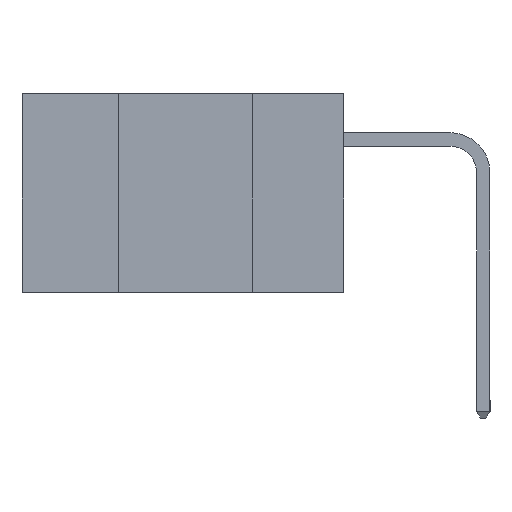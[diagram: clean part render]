
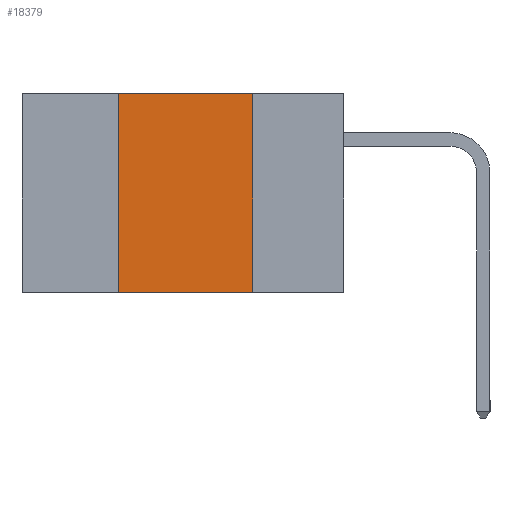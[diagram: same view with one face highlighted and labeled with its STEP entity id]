
A CAD part, left-side view. The second image highlights one B-rep face of the part: STEP entity #18379.
In plain terms, the highlighted planar face has unit normal (-1, 0, 0).
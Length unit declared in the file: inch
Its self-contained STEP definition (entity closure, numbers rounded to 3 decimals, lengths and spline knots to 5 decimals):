
#457 = DIRECTION ( 'NONE',  ( 0., 0., -1. ) ) ;
#1163 = CARTESIAN_POINT ( 'NONE',  ( 0., 0.42, -0.37 ) ) ;
#1395 = CARTESIAN_POINT ( 'NONE',  ( 0., 0.6, 0. ) ) ;
#1983 = ORIENTED_EDGE ( 'NONE', *, *, #7339, .T. ) ;
#4529 = DIRECTION ( 'NONE',  ( 0., -1., 0. ) ) ;
#4716 = DIRECTION ( 'NONE',  ( 0., -1., 0. ) ) ;
#5284 = CARTESIAN_POINT ( 'NONE',  ( 0., 0.6, -0.37 ) ) ;
#5469 = LINE ( 'NONE', #24870, #10307 ) ;
#5555 = ORIENTED_EDGE ( 'NONE', *, *, #8697, .F. ) ;
#6281 = VERTEX_POINT ( 'NONE', #24155 ) ;
#6349 = VERTEX_POINT ( 'NONE', #22588 ) ;
#7238 = FACE_OUTER_BOUND ( 'NONE', #24895, .T. ) ;
#7339 = EDGE_CURVE ( 'NONE', #10685, #6281, #23812, .T. ) ;
#8626 = LINE ( 'NONE', #16956, #13447 ) ;
#8697 = EDGE_CURVE ( 'NONE', #10685, #20961, #18172, .T. ) ;
#10307 = VECTOR ( 'NONE', #4716, 39.37008 ) ;
#10392 = ORIENTED_EDGE ( 'NONE', *, *, #21307, .F. ) ;
#10685 = VERTEX_POINT ( 'NONE', #23984 ) ;
#11809 = DIRECTION ( 'NONE',  ( 0., 0., -1. ) ) ;
#12139 = VECTOR ( 'NONE', #21651, 39.37008 ) ;
#13447 = VECTOR ( 'NONE', #457, 39.37008 ) ;
#16420 = EDGE_CURVE ( 'NONE', #6349, #6281, #8626, .T. ) ;
#16459 = ORIENTED_EDGE ( 'NONE', *, *, #16420, .F. ) ;
#16956 = CARTESIAN_POINT ( 'NONE',  ( 0., 0.17, -0.37 ) ) ;
#18172 = LINE ( 'NONE', #1163, #12139 ) ;
#18379 = ADVANCED_FACE ( 'NONE', ( #7238 ), #21860, .F. ) ;
#18518 = VECTOR ( 'NONE', #4529, 39.37008 ) ;
#20961 = VERTEX_POINT ( 'NONE', #23855 ) ;
#21307 = EDGE_CURVE ( 'NONE', #20961, #6349, #5469, .T. ) ;
#21651 = DIRECTION ( 'NONE',  ( 0., 0., 1. ) ) ;
#21860 = PLANE ( 'NONE',  #24963 ) ;
#22588 = CARTESIAN_POINT ( 'NONE',  ( 0., 0.17, 0. ) ) ;
#23812 = LINE ( 'NONE', #5284, #18518 ) ;
#23844 = DIRECTION ( 'NONE',  ( 1., 0., 0. ) ) ;
#23855 = CARTESIAN_POINT ( 'NONE',  ( 0., 0.42, 0. ) ) ;
#23984 = CARTESIAN_POINT ( 'NONE',  ( 0., 0.42, -0.37 ) ) ;
#24155 = CARTESIAN_POINT ( 'NONE',  ( 0., 0.17, -0.37 ) ) ;
#24870 = CARTESIAN_POINT ( 'NONE',  ( 0., 0.6, 0. ) ) ;
#24895 = EDGE_LOOP ( 'NONE', ( #16459, #10392, #5555, #1983 ) ) ;
#24963 = AXIS2_PLACEMENT_3D ( 'NONE', #1395, #23844, #11809 ) ;
